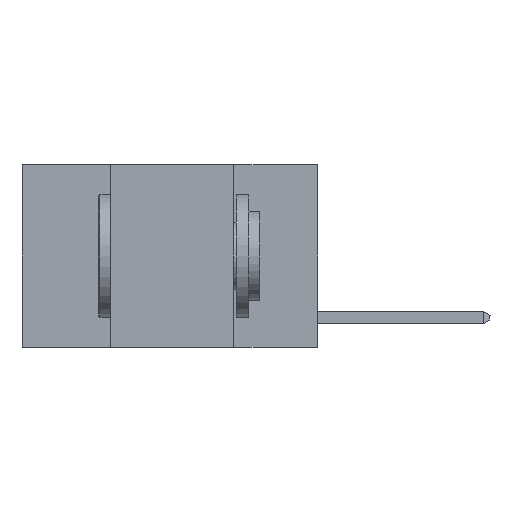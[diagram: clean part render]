
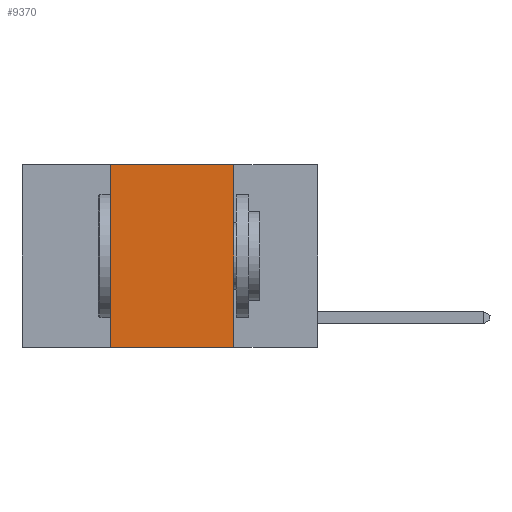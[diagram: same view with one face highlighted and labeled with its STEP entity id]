
A CAD part, left-side view. The second image highlights one B-rep face of the part: STEP entity #9370.
In plain terms, the highlighted planar face has unit normal (-1, 0, 0).
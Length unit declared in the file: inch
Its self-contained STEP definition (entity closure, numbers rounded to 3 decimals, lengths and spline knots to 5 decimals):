
#2507 = ORIENTED_EDGE ( 'NONE', *, *, #27326, .F. ) ;
#2975 = DIRECTION ( 'NONE',  ( 0., 0., 1. ) ) ;
#2977 = CARTESIAN_POINT ( 'NONE',  ( 0., 0.17, 0. ) ) ;
#3621 = CARTESIAN_POINT ( 'NONE',  ( 0., 0.17, -0.37 ) ) ;
#4005 = CARTESIAN_POINT ( 'NONE',  ( 0., 0.42, -0.37 ) ) ;
#6048 = LINE ( 'NONE', #2977, #7300 ) ;
#7300 = VECTOR ( 'NONE', #12008, 39.37008 ) ;
#7553 = EDGE_CURVE ( 'NONE', #11395, #25726, #15579, .T. ) ;
#8444 = CARTESIAN_POINT ( 'NONE',  ( 0., 0.42, 0. ) ) ;
#8689 = DIRECTION ( 'NONE',  ( 0., -1., 0. ) ) ;
#8878 = VECTOR ( 'NONE', #8689, 39.37008 ) ;
#9370 = ADVANCED_FACE ( 'NONE', ( #18635 ), #9433, .F. ) ;
#9433 = PLANE ( 'NONE',  #13806 ) ;
#9560 = VECTOR ( 'NONE', #26513, 39.37008 ) ;
#10288 = ORIENTED_EDGE ( 'NONE', *, *, #7553, .T. ) ;
#10325 = CARTESIAN_POINT ( 'NONE',  ( 0., 0.6, 0. ) ) ;
#11395 = VERTEX_POINT ( 'NONE', #4005 ) ;
#12008 = DIRECTION ( 'NONE',  ( 0., 0., -1. ) ) ;
#12162 = CARTESIAN_POINT ( 'NONE',  ( 0., 0.42, 0. ) ) ;
#13806 = AXIS2_PLACEMENT_3D ( 'NONE', #25143, #24859, #27646 ) ;
#14398 = LINE ( 'NONE', #12162, #19802 ) ;
#15579 = LINE ( 'NONE', #29032, #9560 ) ;
#18635 = FACE_OUTER_BOUND ( 'NONE', #22733, .T. ) ;
#18965 = EDGE_CURVE ( 'NONE', #21003, #28702, #24401, .T. ) ;
#19527 = EDGE_CURVE ( 'NONE', #11395, #21003, #14398, .T. ) ;
#19704 = ORIENTED_EDGE ( 'NONE', *, *, #19527, .F. ) ;
#19802 = VECTOR ( 'NONE', #2975, 39.37008 ) ;
#21003 = VERTEX_POINT ( 'NONE', #8444 ) ;
#22733 = EDGE_LOOP ( 'NONE', ( #2507, #25311, #19704, #10288 ) ) ;
#24401 = LINE ( 'NONE', #10325, #8878 ) ;
#24859 = DIRECTION ( 'NONE',  ( 1., 0., 0. ) ) ;
#25143 = CARTESIAN_POINT ( 'NONE',  ( 0., 0.6, 0. ) ) ;
#25311 = ORIENTED_EDGE ( 'NONE', *, *, #18965, .F. ) ;
#25726 = VERTEX_POINT ( 'NONE', #3621 ) ;
#26212 = CARTESIAN_POINT ( 'NONE',  ( 0., 0.17, 0. ) ) ;
#26513 = DIRECTION ( 'NONE',  ( 0., -1., 0. ) ) ;
#27326 = EDGE_CURVE ( 'NONE', #28702, #25726, #6048, .T. ) ;
#27646 = DIRECTION ( 'NONE',  ( 0., 0., -1. ) ) ;
#28702 = VERTEX_POINT ( 'NONE', #26212 ) ;
#29032 = CARTESIAN_POINT ( 'NONE',  ( 0., 0.6, -0.37 ) ) ;
